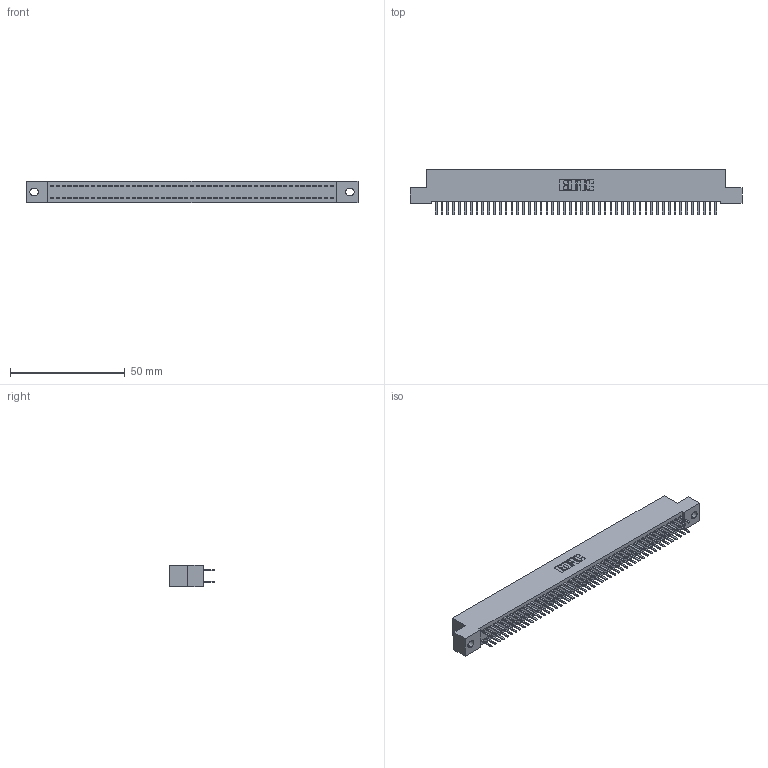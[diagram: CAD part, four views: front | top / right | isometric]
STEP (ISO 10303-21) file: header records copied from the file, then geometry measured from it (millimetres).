
FILE_DESCRIPTION (( 'STEP AP203' ), '1' );
FILE_NAME ('392-098-520-202.STEP', '2019-10-09T20:10:03', ( '' ), ( '' ), 'SwSTEP 2.0', 'SolidWorks 2016', '' );
FILE_SCHEMA (( 'CONFIG_CONTROL_DESIGN' ));
Length unit declared in the file: inch
Products named in the file (3): 392-098-520-202; 342 Part_.128 Slot; 345-292-001_345-293-120
Assembly tree (99 placements, depth 2):
  392-098-520-202
    342 Part_.128 Slot
    345-292-001_345-293-120  x98
Bounding box: 144.78 x 20.02 x 9.4 mm (x, y, z)
Volume: 12946.4 mm3; surface area: 20903.8 mm2
Topology: 99 solids, 99 shells, 5602 faces, 16285 edges, 10594 vertices
Faces by surface type: plane 3794, cylinder 1808
Entity records: 30735 total; most frequent: CARTESIAN_POINT 5098, ORIENTED_EDGE 5022, DIRECTION 4331, EDGE_CURVE 2511, LINE 2379, VECTOR 2379, VERTEX_POINT 1670, AXIS2_PLACEMENT_3D 976
